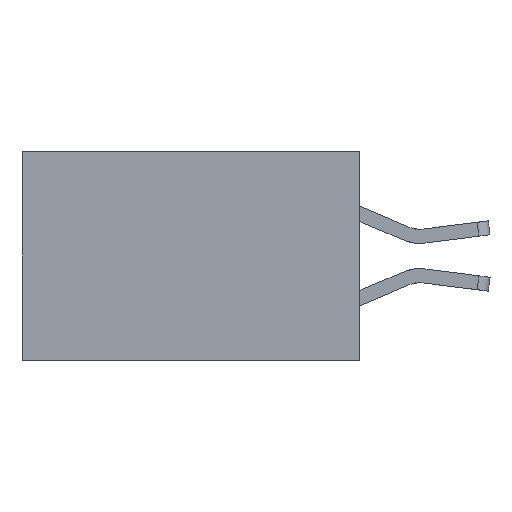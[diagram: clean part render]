
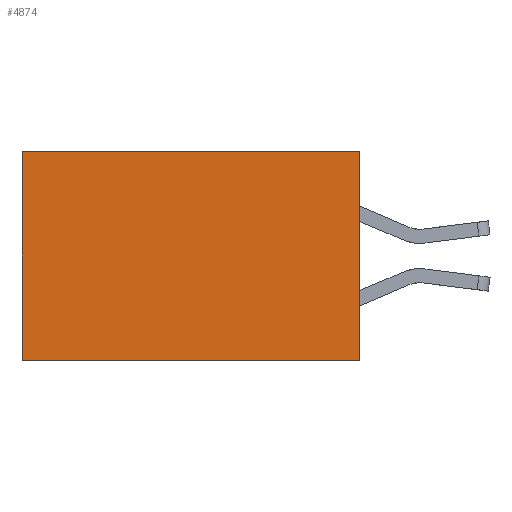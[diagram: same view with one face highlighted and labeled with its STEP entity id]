
A CAD part, left-side view. The second image highlights one B-rep face of the part: STEP entity #4874.
In plain terms, the highlighted planar face has unit normal (-1, 0, 0).
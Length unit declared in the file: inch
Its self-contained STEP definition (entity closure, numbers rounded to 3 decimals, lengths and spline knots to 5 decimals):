
#12 = CARTESIAN_POINT ( 'NONE',  ( 0.2875, 0., 0. ) ) ;
#981 = EDGE_CURVE ( 'NONE', #5485, #9008, #5724, .T. ) ;
#1004 = CARTESIAN_POINT ( 'NONE',  ( 0.2875, 0.6, 0. ) ) ;
#1387 = VECTOR ( 'NONE', #5335, 39.37008 ) ;
#1908 = VECTOR ( 'NONE', #4224, 39.37008 ) ;
#1953 = DIRECTION ( 'NONE',  ( 0., 0., -1. ) ) ;
#2047 = EDGE_LOOP ( 'NONE', ( #4215, #2327, #8764, #3022 ) ) ;
#2247 = CARTESIAN_POINT ( 'NONE',  ( 0.2875, 0., 0. ) ) ;
#2327 = ORIENTED_EDGE ( 'NONE', *, *, #2461, .F. ) ;
#2461 = EDGE_CURVE ( 'NONE', #9008, #7984, #3026, .T. ) ;
#2519 = EDGE_CURVE ( 'NONE', #10411, #7984, #10765, .T. ) ;
#2625 = DIRECTION ( 'NONE',  ( 1., 0., 0. ) ) ;
#3022 = ORIENTED_EDGE ( 'NONE', *, *, #8106, .T. ) ;
#3026 = LINE ( 'NONE', #8321, #5042 ) ;
#4215 = ORIENTED_EDGE ( 'NONE', *, *, #2519, .T. ) ;
#4224 = DIRECTION ( 'NONE',  ( 0., 0., -1. ) ) ;
#4472 = PLANE ( 'NONE',  #6301 ) ;
#4874 = ADVANCED_FACE ( 'NONE', ( #10461 ), #4472, .F. ) ;
#4891 = CARTESIAN_POINT ( 'NONE',  ( 0.2875, 0., 0. ) ) ;
#4986 = CARTESIAN_POINT ( 'NONE',  ( 0.2875, 0., 0. ) ) ;
#5042 = VECTOR ( 'NONE', #8140, 39.37008 ) ;
#5280 = CARTESIAN_POINT ( 'NONE',  ( 0.2875, 0.6, 0. ) ) ;
#5335 = DIRECTION ( 'NONE',  ( 0., 0., -1. ) ) ;
#5485 = VERTEX_POINT ( 'NONE', #4986 ) ;
#5724 = LINE ( 'NONE', #4891, #1387 ) ;
#6301 = AXIS2_PLACEMENT_3D ( 'NONE', #2247, #2625, #1953 ) ;
#6536 = CARTESIAN_POINT ( 'NONE',  ( 0.2875, 0., -0.37 ) ) ;
#6799 = CARTESIAN_POINT ( 'NONE',  ( 0.2875, 0.6, -0.37 ) ) ;
#6870 = VECTOR ( 'NONE', #9362, 39.37008 ) ;
#7984 = VERTEX_POINT ( 'NONE', #6799 ) ;
#8106 = EDGE_CURVE ( 'NONE', #5485, #10411, #9265, .T. ) ;
#8140 = DIRECTION ( 'NONE',  ( 0., 1., 0. ) ) ;
#8321 = CARTESIAN_POINT ( 'NONE',  ( 0.2875, 0., -0.37 ) ) ;
#8764 = ORIENTED_EDGE ( 'NONE', *, *, #981, .F. ) ;
#9008 = VERTEX_POINT ( 'NONE', #6536 ) ;
#9265 = LINE ( 'NONE', #12, #6870 ) ;
#9362 = DIRECTION ( 'NONE',  ( 0., 1., 0. ) ) ;
#10411 = VERTEX_POINT ( 'NONE', #5280 ) ;
#10461 = FACE_OUTER_BOUND ( 'NONE', #2047, .T. ) ;
#10765 = LINE ( 'NONE', #1004, #1908 ) ;
